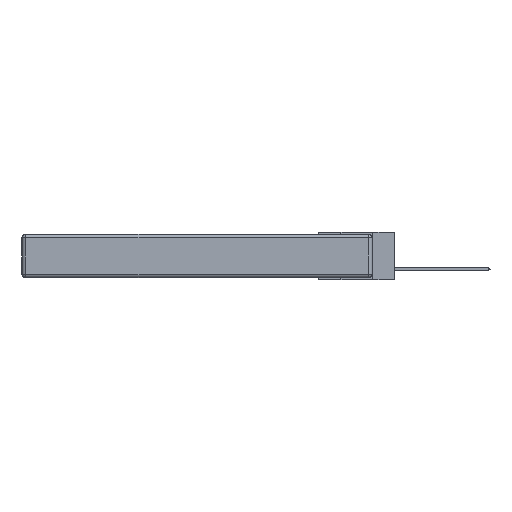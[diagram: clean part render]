
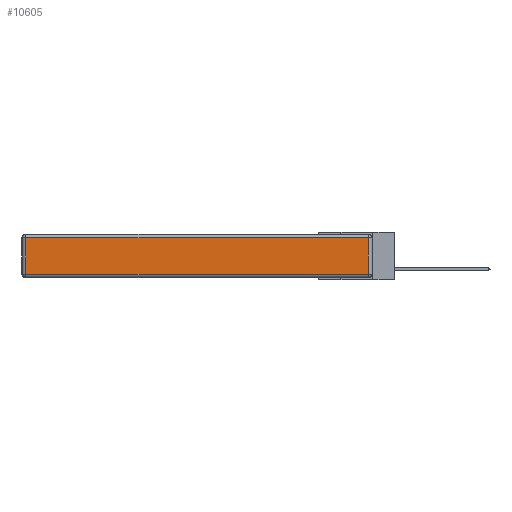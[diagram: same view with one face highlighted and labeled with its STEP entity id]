
A CAD part, left-side view. The second image highlights one B-rep face of the part: STEP entity #10605.
In plain terms, the highlighted planar face has unit normal (-1, 0, 0).
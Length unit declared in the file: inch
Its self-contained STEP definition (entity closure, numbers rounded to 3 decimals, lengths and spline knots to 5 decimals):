
#869 = DIRECTION ( 'NONE',  ( 0., -1., 0. ) ) ;
#1553 = CARTESIAN_POINT ( 'NONE',  ( 0., 0.03, -0.313 ) ) ;
#2184 = DIRECTION ( 'NONE',  ( 0., 0., 1. ) ) ;
#2238 = VERTEX_POINT ( 'NONE', #15665 ) ;
#4006 = VECTOR ( 'NONE', #869, 39.37008 ) ;
#4323 = LINE ( 'NONE', #21510, #23578 ) ;
#4470 = CARTESIAN_POINT ( 'NONE',  ( 0., 0., -0.313 ) ) ;
#5054 = LINE ( 'NONE', #20880, #22573 ) ;
#5277 = CARTESIAN_POINT ( 'NONE',  ( 0., 0., -0.343 ) ) ;
#6444 = EDGE_CURVE ( 'NONE', #2238, #14594, #4323, .T. ) ;
#6591 = ORIENTED_EDGE ( 'NONE', *, *, #16778, .T. ) ;
#8642 = EDGE_CURVE ( 'NONE', #14545, #2238, #15677, .T. ) ;
#10421 = CARTESIAN_POINT ( 'NONE',  ( 0., 2.75, -0.03 ) ) ;
#10605 = ADVANCED_FACE ( 'NONE', ( #16934 ), #22186, .T. ) ;
#10690 = VECTOR ( 'NONE', #17836, 39.37008 ) ;
#11020 = LINE ( 'NONE', #4470, #4006 ) ;
#11035 = CARTESIAN_POINT ( 'NONE',  ( 0., 2.72, -0.313 ) ) ;
#11796 = ORIENTED_EDGE ( 'NONE', *, *, #6444, .T. ) ;
#12535 = ORIENTED_EDGE ( 'NONE', *, *, #8642, .T. ) ;
#12568 = DIRECTION ( 'NONE',  ( 0., 0., 1. ) ) ;
#14545 = VERTEX_POINT ( 'NONE', #18213 ) ;
#14594 = VERTEX_POINT ( 'NONE', #11035 ) ;
#15665 = CARTESIAN_POINT ( 'NONE',  ( 0., 2.72, -0.03 ) ) ;
#15677 = LINE ( 'NONE', #10421, #10690 ) ;
#15804 = DIRECTION ( 'NONE',  ( 0., 0., -1. ) ) ;
#16778 = EDGE_CURVE ( 'NONE', #14594, #17507, #11020, .T. ) ;
#16934 = FACE_OUTER_BOUND ( 'NONE', #23816, .T. ) ;
#17507 = VERTEX_POINT ( 'NONE', #1553 ) ;
#17836 = DIRECTION ( 'NONE',  ( 0., 1., 0. ) ) ;
#18179 = ORIENTED_EDGE ( 'NONE', *, *, #23344, .T. ) ;
#18213 = CARTESIAN_POINT ( 'NONE',  ( 0., 0.03, -0.03 ) ) ;
#19250 = AXIS2_PLACEMENT_3D ( 'NONE', #5277, #20227, #12568 ) ;
#20227 = DIRECTION ( 'NONE',  ( -1., 0., 0. ) ) ;
#20880 = CARTESIAN_POINT ( 'NONE',  ( 0., 0.03, -0.343 ) ) ;
#21510 = CARTESIAN_POINT ( 'NONE',  ( 0., 2.72, -0.343 ) ) ;
#22186 = PLANE ( 'NONE',  #19250 ) ;
#22573 = VECTOR ( 'NONE', #2184, 39.37008 ) ;
#23344 = EDGE_CURVE ( 'NONE', #17507, #14545, #5054, .T. ) ;
#23578 = VECTOR ( 'NONE', #15804, 39.37008 ) ;
#23816 = EDGE_LOOP ( 'NONE', ( #6591, #18179, #12535, #11796 ) ) ;
